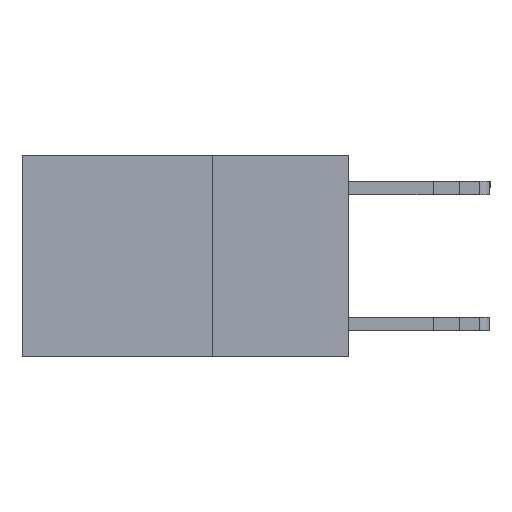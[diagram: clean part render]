
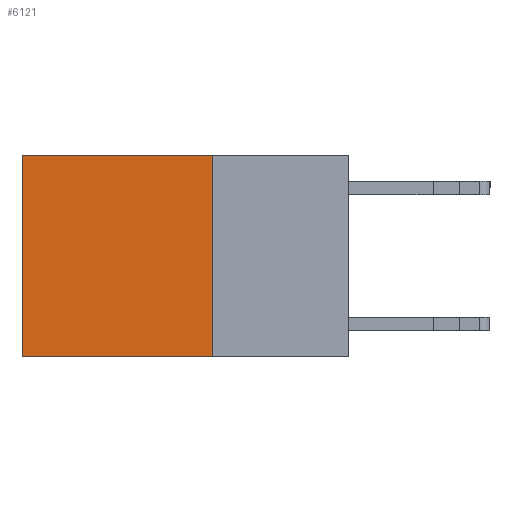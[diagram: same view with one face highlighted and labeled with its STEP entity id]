
A CAD part, left-side view. The second image highlights one B-rep face of the part: STEP entity #6121.
In plain terms, the highlighted planar face has unit normal (-1, 0, 0).
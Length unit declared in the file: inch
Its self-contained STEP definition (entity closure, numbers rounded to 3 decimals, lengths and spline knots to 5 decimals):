
#44 = CARTESIAN_POINT ( 'NONE',  ( 0.2625, 0.25, 0. ) ) ;
#359 = CARTESIAN_POINT ( 'NONE',  ( 0.2625, 0.25, 0. ) ) ;
#450 = CARTESIAN_POINT ( 'NONE',  ( 0.2625, 0.6, 0. ) ) ;
#972 = LINE ( 'NONE', #4687, #1176 ) ;
#1176 = VECTOR ( 'NONE', #12278, 39.37008 ) ;
#1375 = ORIENTED_EDGE ( 'NONE', *, *, #12526, .F. ) ;
#1583 = AXIS2_PLACEMENT_3D ( 'NONE', #10992, #2347, #5012 ) ;
#1646 = LINE ( 'NONE', #450, #15523 ) ;
#2347 = DIRECTION ( 'NONE',  ( 1., 0., 0. ) ) ;
#2641 = VERTEX_POINT ( 'NONE', #15276 ) ;
#2969 = DIRECTION ( 'NONE',  ( 0., 0., -1. ) ) ;
#3556 = EDGE_CURVE ( 'NONE', #8383, #4513, #8938, .T. ) ;
#3606 = EDGE_CURVE ( 'NONE', #4513, #12339, #1646, .T. ) ;
#4513 = VERTEX_POINT ( 'NONE', #10358 ) ;
#4687 = CARTESIAN_POINT ( 'NONE',  ( 0.2625, 0.25, -0.37 ) ) ;
#5012 = DIRECTION ( 'NONE',  ( 0., 0., -1. ) ) ;
#5630 = LINE ( 'NONE', #10550, #10216 ) ;
#5979 = PLANE ( 'NONE',  #1583 ) ;
#6121 = ADVANCED_FACE ( 'NONE', ( #7495 ), #5979, .F. ) ;
#6477 = VECTOR ( 'NONE', #7543, 39.37008 ) ;
#6826 = DIRECTION ( 'NONE',  ( 0., 0., -1. ) ) ;
#7084 = ORIENTED_EDGE ( 'NONE', *, *, #3606, .T. ) ;
#7495 = FACE_OUTER_BOUND ( 'NONE', #8369, .T. ) ;
#7543 = DIRECTION ( 'NONE',  ( 0., 1., 0. ) ) ;
#8369 = EDGE_LOOP ( 'NONE', ( #7084, #1375, #8486, #10537 ) ) ;
#8383 = VERTEX_POINT ( 'NONE', #359 ) ;
#8486 = ORIENTED_EDGE ( 'NONE', *, *, #11894, .F. ) ;
#8938 = LINE ( 'NONE', #44, #6477 ) ;
#9553 = CARTESIAN_POINT ( 'NONE',  ( 0.2625, 0.6, -0.37 ) ) ;
#10216 = VECTOR ( 'NONE', #2969, 39.37008 ) ;
#10358 = CARTESIAN_POINT ( 'NONE',  ( 0.2625, 0.6, 0. ) ) ;
#10537 = ORIENTED_EDGE ( 'NONE', *, *, #3556, .T. ) ;
#10550 = CARTESIAN_POINT ( 'NONE',  ( 0.2625, 0.25, 0. ) ) ;
#10992 = CARTESIAN_POINT ( 'NONE',  ( 0.2625, 0.25, 0. ) ) ;
#11894 = EDGE_CURVE ( 'NONE', #8383, #2641, #5630, .T. ) ;
#12278 = DIRECTION ( 'NONE',  ( 0., 1., 0. ) ) ;
#12339 = VERTEX_POINT ( 'NONE', #9553 ) ;
#12526 = EDGE_CURVE ( 'NONE', #2641, #12339, #972, .T. ) ;
#15276 = CARTESIAN_POINT ( 'NONE',  ( 0.2625, 0.25, -0.37 ) ) ;
#15523 = VECTOR ( 'NONE', #6826, 39.37008 ) ;
